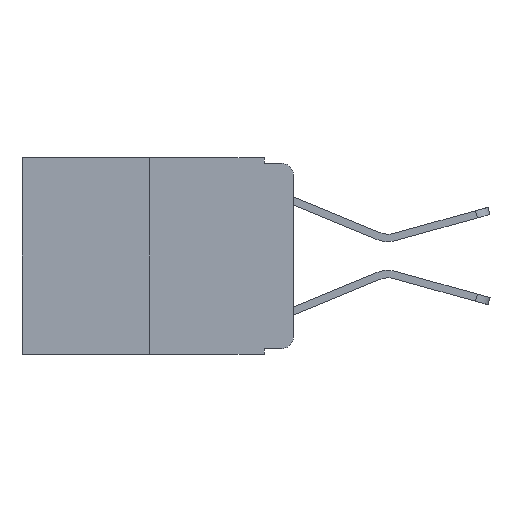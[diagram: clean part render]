
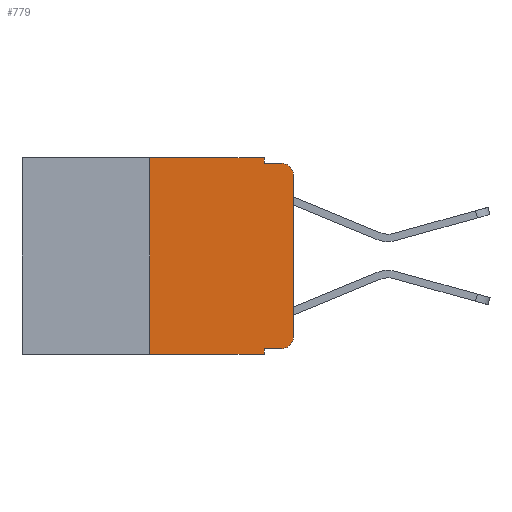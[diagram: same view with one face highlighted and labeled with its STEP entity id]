
A CAD part, left-side view. The second image highlights one B-rep face of the part: STEP entity #779.
In plain terms, the highlighted planar face has unit normal (-1, 0, 0).
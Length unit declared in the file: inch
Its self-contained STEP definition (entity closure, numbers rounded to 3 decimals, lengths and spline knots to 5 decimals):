
#423 = VECTOR ( 'NONE', #10461, 39.37008 ) ;
#601 = VECTOR ( 'NONE', #15130, 39.37008 ) ;
#619 = VERTEX_POINT ( 'NONE', #11308 ) ;
#655 = ORIENTED_EDGE ( 'NONE', *, *, #10445, .F. ) ;
#779 = ADVANCED_FACE ( 'NONE', ( #5953 ), #5357, .F. ) ;
#1701 = VECTOR ( 'NONE', #20526, 39.37008 ) ;
#2031 = CARTESIAN_POINT ( 'NONE',  ( 0., 0.02, -0.313 ) ) ;
#2116 = VERTEX_POINT ( 'NONE', #17998 ) ;
#2118 = LINE ( 'NONE', #16798, #11391 ) ;
#2455 = LINE ( 'NONE', #14078, #1701 ) ;
#2488 = ORIENTED_EDGE ( 'NONE', *, *, #19925, .F. ) ;
#2734 = CARTESIAN_POINT ( 'NONE',  ( 0., 0.02, -0.03 ) ) ;
#3221 = VERTEX_POINT ( 'NONE', #10193 ) ;
#3843 = LINE ( 'NONE', #8759, #13650 ) ;
#4492 = LINE ( 'NONE', #16373, #18212 ) ;
#4767 = LINE ( 'NONE', #10683, #423 ) ;
#4832 = DIRECTION ( 'NONE',  ( 0., 0., -1. ) ) ;
#5022 = DIRECTION ( 'NONE',  ( -1., 0., 0. ) ) ;
#5138 = CARTESIAN_POINT ( 'NONE',  ( 0., 0.25, 0. ) ) ;
#5192 = EDGE_CURVE ( 'NONE', #3221, #6141, #19516, .T. ) ;
#5357 = PLANE ( 'NONE',  #14808 ) ;
#5439 = EDGE_CURVE ( 'NONE', #6543, #13219, #4492, .T. ) ;
#5873 = DIRECTION ( 'NONE',  ( 0., 0., 1. ) ) ;
#5922 = ORIENTED_EDGE ( 'NONE', *, *, #5439, .F. ) ;
#5944 = ORIENTED_EDGE ( 'NONE', *, *, #13152, .F. ) ;
#5953 = FACE_OUTER_BOUND ( 'NONE', #21042, .T. ) ;
#6141 = VERTEX_POINT ( 'NONE', #18466 ) ;
#6543 = VERTEX_POINT ( 'NONE', #14700 ) ;
#6799 = ORIENTED_EDGE ( 'NONE', *, *, #14989, .T. ) ;
#7100 = DIRECTION ( 'NONE',  ( 0., 0., -1. ) ) ;
#7152 = VERTEX_POINT ( 'NONE', #16826 ) ;
#7713 = CARTESIAN_POINT ( 'NONE',  ( 0., 0.051, -0.343 ) ) ;
#8476 = AXIS2_PLACEMENT_3D ( 'NONE', #2734, #17578, #10913 ) ;
#8646 = VECTOR ( 'NONE', #5873, 39.37008 ) ;
#8759 = CARTESIAN_POINT ( 'NONE',  ( 0., 0.051, 0. ) ) ;
#8982 = EDGE_CURVE ( 'NONE', #7152, #6543, #2455, .T. ) ;
#9054 = CARTESIAN_POINT ( 'NONE',  ( 0., 0., 0. ) ) ;
#10193 = CARTESIAN_POINT ( 'NONE',  ( 0., 0., -0.03 ) ) ;
#10372 = LINE ( 'NONE', #5138, #601 ) ;
#10445 = EDGE_CURVE ( 'NONE', #619, #7152, #10372, .T. ) ;
#10461 = DIRECTION ( 'NONE',  ( 0., -1., 0. ) ) ;
#10683 = CARTESIAN_POINT ( 'NONE',  ( 0., 0.473, -0.343 ) ) ;
#10913 = DIRECTION ( 'NONE',  ( 0., 0., -1. ) ) ;
#10928 = DIRECTION ( 'NONE',  ( 0., -1., 0. ) ) ;
#11308 = CARTESIAN_POINT ( 'NONE',  ( 0., 0.25, -0.343 ) ) ;
#11381 = EDGE_CURVE ( 'NONE', #17062, #2116, #13436, .T. ) ;
#11391 = VECTOR ( 'NONE', #20136, 39.37008 ) ;
#12153 = DIRECTION ( 'NONE',  ( 1., 0., 0. ) ) ;
#12421 = VECTOR ( 'NONE', #10928, 39.37008 ) ;
#12951 = ORIENTED_EDGE ( 'NONE', *, *, #5192, .T. ) ;
#13152 = EDGE_CURVE ( 'NONE', #14030, #16565, #3843, .T. ) ;
#13216 = LINE ( 'NONE', #20724, #12421 ) ;
#13219 = VERTEX_POINT ( 'NONE', #14062 ) ;
#13436 = CIRCLE ( 'NONE', #13536, 0.02 ) ;
#13536 = AXIS2_PLACEMENT_3D ( 'NONE', #2031, #5022, #18259 ) ;
#13650 = VECTOR ( 'NONE', #20373, 39.37008 ) ;
#14030 = VERTEX_POINT ( 'NONE', #16524 ) ;
#14062 = CARTESIAN_POINT ( 'NONE',  ( 0., 0.051, -0.01 ) ) ;
#14078 = CARTESIAN_POINT ( 'NONE',  ( 0., 0.473, 0. ) ) ;
#14700 = CARTESIAN_POINT ( 'NONE',  ( 0., 0.051, 0. ) ) ;
#14808 = AXIS2_PLACEMENT_3D ( 'NONE', #18669, #12153, #7100 ) ;
#14989 = EDGE_CURVE ( 'NONE', #2116, #3221, #16720, .T. ) ;
#15130 = DIRECTION ( 'NONE',  ( 0., 0., 1. ) ) ;
#16373 = CARTESIAN_POINT ( 'NONE',  ( 0., 0.051, 0. ) ) ;
#16414 = EDGE_CURVE ( 'NONE', #619, #16565, #4767, .T. ) ;
#16425 = ORIENTED_EDGE ( 'NONE', *, *, #8982, .F. ) ;
#16524 = CARTESIAN_POINT ( 'NONE',  ( 0., 0.051, -0.333 ) ) ;
#16565 = VERTEX_POINT ( 'NONE', #7713 ) ;
#16720 = LINE ( 'NONE', #9054, #8646 ) ;
#16798 = CARTESIAN_POINT ( 'NONE',  ( 0., 0.051, -0.333 ) ) ;
#16826 = CARTESIAN_POINT ( 'NONE',  ( 0., 0.25, 0. ) ) ;
#16910 = ORIENTED_EDGE ( 'NONE', *, *, #20304, .T. ) ;
#17062 = VERTEX_POINT ( 'NONE', #18768 ) ;
#17147 = ORIENTED_EDGE ( 'NONE', *, *, #11381, .T. ) ;
#17578 = DIRECTION ( 'NONE',  ( -1., 0., 0. ) ) ;
#17998 = CARTESIAN_POINT ( 'NONE',  ( 0., 0., -0.313 ) ) ;
#18212 = VECTOR ( 'NONE', #4832, 39.37008 ) ;
#18259 = DIRECTION ( 'NONE',  ( 0., 0., -1. ) ) ;
#18466 = CARTESIAN_POINT ( 'NONE',  ( 0., 0.02, -0.01 ) ) ;
#18669 = CARTESIAN_POINT ( 'NONE',  ( 0., 0.473, 0. ) ) ;
#18768 = CARTESIAN_POINT ( 'NONE',  ( 0., 0.02, -0.333 ) ) ;
#19516 = CIRCLE ( 'NONE', #8476, 0.02 ) ;
#19925 = EDGE_CURVE ( 'NONE', #13219, #6141, #13216, .T. ) ;
#20136 = DIRECTION ( 'NONE',  ( 0., -1., 0. ) ) ;
#20304 = EDGE_CURVE ( 'NONE', #14030, #17062, #2118, .T. ) ;
#20373 = DIRECTION ( 'NONE',  ( 0., 0., -1. ) ) ;
#20526 = DIRECTION ( 'NONE',  ( 0., -1., 0. ) ) ;
#20724 = CARTESIAN_POINT ( 'NONE',  ( 0., 0.051, -0.01 ) ) ;
#21042 = EDGE_LOOP ( 'NONE', ( #6799, #12951, #2488, #5922, #16425, #655, #21291, #5944, #16910, #17147 ) ) ;
#21291 = ORIENTED_EDGE ( 'NONE', *, *, #16414, .T. ) ;
